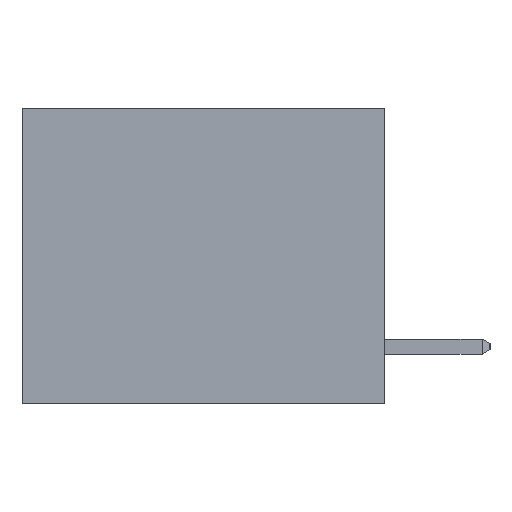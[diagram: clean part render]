
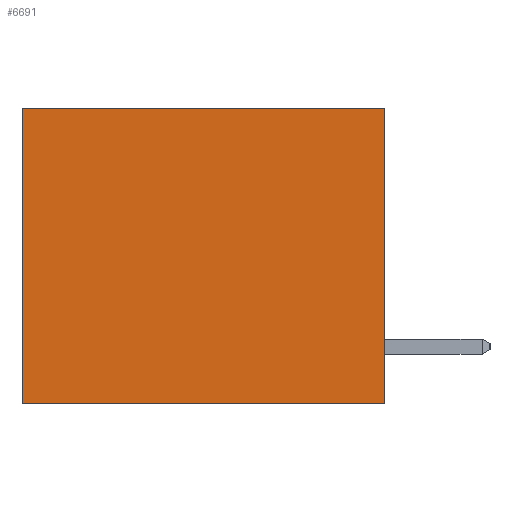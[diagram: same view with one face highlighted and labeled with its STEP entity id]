
A CAD part, left-side view. The second image highlights one B-rep face of the part: STEP entity #6691.
In plain terms, the highlighted planar face has unit normal (-1, 0, 0).
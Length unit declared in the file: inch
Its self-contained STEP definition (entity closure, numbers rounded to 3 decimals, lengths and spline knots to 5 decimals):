
#785 = ORIENTED_EDGE ( 'NONE', *, *, #12955, .F. ) ;
#2176 = CARTESIAN_POINT ( 'NONE',  ( 0.3165, 0., -0.49 ) ) ;
#2397 = EDGE_CURVE ( 'NONE', #16072, #3490, #21176, .T. ) ;
#3490 = VERTEX_POINT ( 'NONE', #18610 ) ;
#3910 = VECTOR ( 'NONE', #11570, 39.37008 ) ;
#3948 = DIRECTION ( 'NONE',  ( 0., 1., 0. ) ) ;
#4067 = AXIS2_PLACEMENT_3D ( 'NONE', #2176, #15924, #5746 ) ;
#5733 = ORIENTED_EDGE ( 'NONE', *, *, #2397, .T. ) ;
#5746 = DIRECTION ( 'NONE',  ( 0., 0., -1. ) ) ;
#6195 = DIRECTION ( 'NONE',  ( 0., 0., -1. ) ) ;
#6691 = ADVANCED_FACE ( 'NONE', ( #9625 ), #12498, .F. ) ;
#6987 = CARTESIAN_POINT ( 'NONE',  ( 0.3165, 0., 0. ) ) ;
#7055 = CARTESIAN_POINT ( 'NONE',  ( 0.3165, 0., -0.49 ) ) ;
#7072 = VERTEX_POINT ( 'NONE', #13404 ) ;
#7514 = ORIENTED_EDGE ( 'NONE', *, *, #11980, .T. ) ;
#7920 = EDGE_CURVE ( 'NONE', #12280, #3490, #16230, .T. ) ;
#7980 = VECTOR ( 'NONE', #3948, 39.37008 ) ;
#9559 = ORIENTED_EDGE ( 'NONE', *, *, #7920, .F. ) ;
#9625 = FACE_OUTER_BOUND ( 'NONE', #19353, .T. ) ;
#9789 = LINE ( 'NONE', #11240, #12411 ) ;
#10711 = VECTOR ( 'NONE', #20308, 39.37008 ) ;
#11240 = CARTESIAN_POINT ( 'NONE',  ( 0.3165, 0., -0.49 ) ) ;
#11570 = DIRECTION ( 'NONE',  ( 0., 0., -1. ) ) ;
#11980 = EDGE_CURVE ( 'NONE', #7072, #16072, #19762, .T. ) ;
#12034 = CARTESIAN_POINT ( 'NONE',  ( 0.3165, 0.6, 0. ) ) ;
#12280 = VERTEX_POINT ( 'NONE', #15256 ) ;
#12411 = VECTOR ( 'NONE', #6195, 39.37008 ) ;
#12498 = PLANE ( 'NONE',  #4067 ) ;
#12955 = EDGE_CURVE ( 'NONE', #7072, #12280, #9789, .T. ) ;
#13404 = CARTESIAN_POINT ( 'NONE',  ( 0.3165, 0., 0. ) ) ;
#15256 = CARTESIAN_POINT ( 'NONE',  ( 0.3165, 0., -0.49 ) ) ;
#15924 = DIRECTION ( 'NONE',  ( 1., 0., 0. ) ) ;
#16072 = VERTEX_POINT ( 'NONE', #12034 ) ;
#16230 = LINE ( 'NONE', #7055, #7980 ) ;
#16623 = CARTESIAN_POINT ( 'NONE',  ( 0.3165, 0.6, -0.49 ) ) ;
#18610 = CARTESIAN_POINT ( 'NONE',  ( 0.3165, 0.6, -0.49 ) ) ;
#19353 = EDGE_LOOP ( 'NONE', ( #5733, #9559, #785, #7514 ) ) ;
#19762 = LINE ( 'NONE', #6987, #10711 ) ;
#20308 = DIRECTION ( 'NONE',  ( 0., 1., 0. ) ) ;
#21176 = LINE ( 'NONE', #16623, #3910 ) ;
